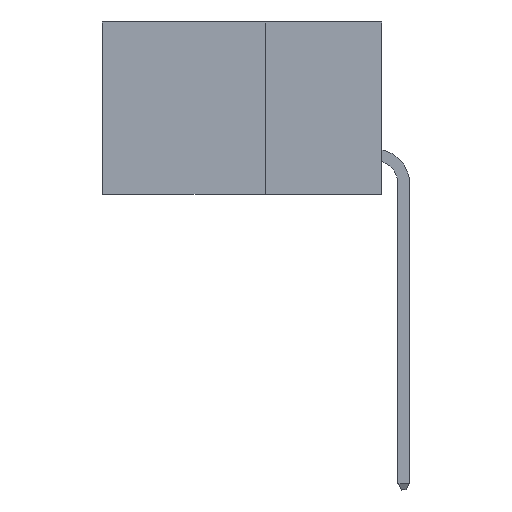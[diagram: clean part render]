
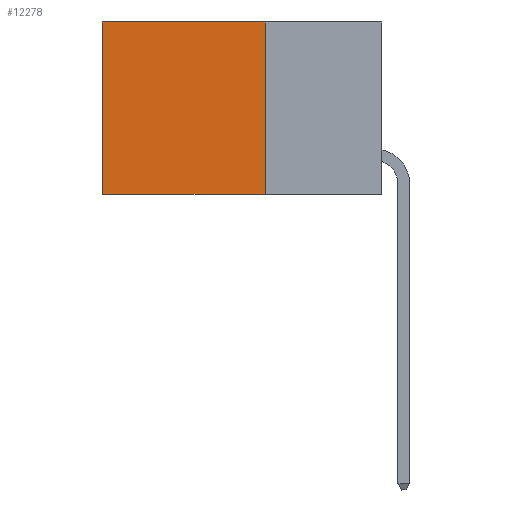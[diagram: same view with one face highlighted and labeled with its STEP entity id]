
A CAD part, left-side view. The second image highlights one B-rep face of the part: STEP entity #12278.
In plain terms, the highlighted planar face has unit normal (-1, 0, 0).
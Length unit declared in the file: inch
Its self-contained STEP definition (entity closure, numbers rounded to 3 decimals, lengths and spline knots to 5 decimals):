
#391 = DIRECTION ( 'NONE',  ( 0., 0., -1. ) ) ;
#414 = CARTESIAN_POINT ( 'NONE',  ( 0.2875, 0.25, -0.37 ) ) ;
#2018 = DIRECTION ( 'NONE',  ( 1., 0., 0. ) ) ;
#2866 = LINE ( 'NONE', #11271, #4452 ) ;
#4452 = VECTOR ( 'NONE', #16724, 39.37008 ) ;
#7039 = VECTOR ( 'NONE', #19100, 39.37008 ) ;
#7317 = CARTESIAN_POINT ( 'NONE',  ( 0.2875, 0.25, 0. ) ) ;
#8045 = ORIENTED_EDGE ( 'NONE', *, *, #30943, .F. ) ;
#8290 = CARTESIAN_POINT ( 'NONE',  ( 0.2875, 0.25, 0. ) ) ;
#9777 = LINE ( 'NONE', #31362, #7039 ) ;
#10340 = EDGE_CURVE ( 'NONE', #15041, #24569, #10855, .T. ) ;
#10855 = LINE ( 'NONE', #8290, #29967 ) ;
#11271 = CARTESIAN_POINT ( 'NONE',  ( 0.2875, 0.25, -0.37 ) ) ;
#12278 = ADVANCED_FACE ( 'NONE', ( #14312 ), #27339, .F. ) ;
#14095 = ORIENTED_EDGE ( 'NONE', *, *, #10340, .T. ) ;
#14312 = FACE_OUTER_BOUND ( 'NONE', #18880, .T. ) ;
#15041 = VERTEX_POINT ( 'NONE', #15467 ) ;
#15467 = CARTESIAN_POINT ( 'NONE',  ( 0.2875, 0.25, 0. ) ) ;
#16724 = DIRECTION ( 'NONE',  ( 0., 1., 0. ) ) ;
#16858 = EDGE_CURVE ( 'NONE', #24569, #26644, #29759, .T. ) ;
#17188 = CARTESIAN_POINT ( 'NONE',  ( 0.2875, 0.6, -0.37 ) ) ;
#18458 = EDGE_CURVE ( 'NONE', #15041, #20512, #9777, .T. ) ;
#18504 = AXIS2_PLACEMENT_3D ( 'NONE', #7317, #2018, #32230 ) ;
#18880 = EDGE_LOOP ( 'NONE', ( #24954, #8045, #28791, #14095 ) ) ;
#19100 = DIRECTION ( 'NONE',  ( 0., 0., -1. ) ) ;
#20512 = VERTEX_POINT ( 'NONE', #414 ) ;
#21575 = VECTOR ( 'NONE', #391, 39.37008 ) ;
#23952 = DIRECTION ( 'NONE',  ( 0., 1., 0. ) ) ;
#24188 = CARTESIAN_POINT ( 'NONE',  ( 0.2875, 0.6, 0. ) ) ;
#24569 = VERTEX_POINT ( 'NONE', #24188 ) ;
#24954 = ORIENTED_EDGE ( 'NONE', *, *, #16858, .T. ) ;
#26644 = VERTEX_POINT ( 'NONE', #17188 ) ;
#27339 = PLANE ( 'NONE',  #18504 ) ;
#27814 = CARTESIAN_POINT ( 'NONE',  ( 0.2875, 0.6, 0. ) ) ;
#28791 = ORIENTED_EDGE ( 'NONE', *, *, #18458, .F. ) ;
#29759 = LINE ( 'NONE', #27814, #21575 ) ;
#29967 = VECTOR ( 'NONE', #23952, 39.37008 ) ;
#30943 = EDGE_CURVE ( 'NONE', #20512, #26644, #2866, .T. ) ;
#31362 = CARTESIAN_POINT ( 'NONE',  ( 0.2875, 0.25, 0. ) ) ;
#32230 = DIRECTION ( 'NONE',  ( 0., 0., -1. ) ) ;
